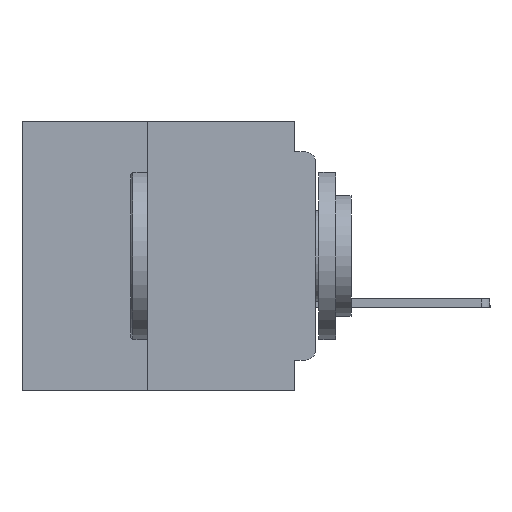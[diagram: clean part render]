
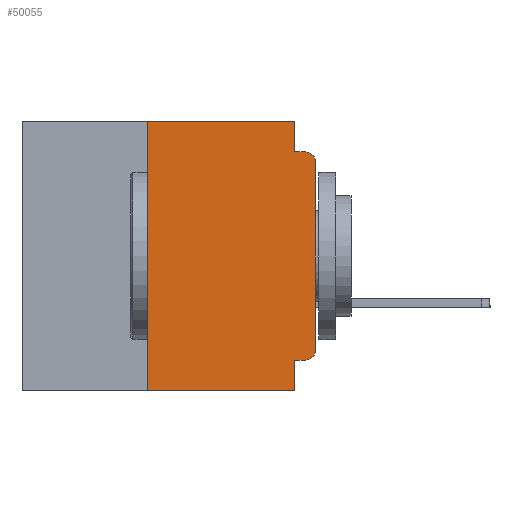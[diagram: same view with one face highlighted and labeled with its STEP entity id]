
A CAD part, left-side view. The second image highlights one B-rep face of the part: STEP entity #50055.
In plain terms, the highlighted planar face has unit normal (-1, 0, 0).
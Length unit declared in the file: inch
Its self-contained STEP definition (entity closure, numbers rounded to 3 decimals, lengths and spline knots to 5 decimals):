
#32 = DIRECTION ( 'NONE',  ( 0., -1., 0. ) ) ;
#233 = CARTESIAN_POINT ( 'NONE',  ( 0., 0.031, -0.4 ) ) ;
#2347 = CARTESIAN_POINT ( 'NONE',  ( 0., 0.437, 0. ) ) ;
#2412 = ORIENTED_EDGE ( 'NONE', *, *, #21963, .F. ) ;
#2658 = VERTEX_POINT ( 'NONE', #31188 ) ;
#2677 = CARTESIAN_POINT ( 'NONE',  ( 0., 0.031, -0.045 ) ) ;
#3046 = CARTESIAN_POINT ( 'NONE',  ( 0., 0.015, -0.355 ) ) ;
#3271 = CARTESIAN_POINT ( 'NONE',  ( 0., 0.437, -0.4 ) ) ;
#3938 = CARTESIAN_POINT ( 'NONE',  ( 0., 0.437, 0. ) ) ;
#4752 = CIRCLE ( 'NONE', #21019, 0.015 ) ;
#5465 = CARTESIAN_POINT ( 'NONE',  ( 0., 0., -0.06 ) ) ;
#7526 = DIRECTION ( 'NONE',  ( 0., -1., 0. ) ) ;
#7736 = CARTESIAN_POINT ( 'NONE',  ( 0., 0.031, 0. ) ) ;
#8598 = EDGE_CURVE ( 'NONE', #13141, #32965, #4752, .T. ) ;
#10267 = DIRECTION ( 'NONE',  ( -1., 0., 0. ) ) ;
#10346 = VECTOR ( 'NONE', #43938, 39.37008 ) ;
#10355 = ORIENTED_EDGE ( 'NONE', *, *, #50103, .F. ) ;
#10613 = ORIENTED_EDGE ( 'NONE', *, *, #42960, .T. ) ;
#11469 = LINE ( 'NONE', #14997, #44432 ) ;
#12647 = ORIENTED_EDGE ( 'NONE', *, *, #53464, .F. ) ;
#12721 = ORIENTED_EDGE ( 'NONE', *, *, #18864, .T. ) ;
#13141 = VERTEX_POINT ( 'NONE', #5465 ) ;
#14222 = VECTOR ( 'NONE', #24063, 39.37008 ) ;
#14935 = LINE ( 'NONE', #7736, #45246 ) ;
#14997 = CARTESIAN_POINT ( 'NONE',  ( 0., 0., 0. ) ) ;
#15523 = VECTOR ( 'NONE', #32, 39.37008 ) ;
#15670 = CARTESIAN_POINT ( 'NONE',  ( 0., 0.031, -0.4 ) ) ;
#16669 = DIRECTION ( 'NONE',  ( 1., 0., 0. ) ) ;
#17147 = DIRECTION ( 'NONE',  ( 0., 0., 1. ) ) ;
#17294 = VERTEX_POINT ( 'NONE', #37693 ) ;
#18864 = EDGE_CURVE ( 'NONE', #2658, #13141, #11469, .T. ) ;
#18992 = VERTEX_POINT ( 'NONE', #19981 ) ;
#19160 = CARTESIAN_POINT ( 'NONE',  ( 0., 0.25, -0.4 ) ) ;
#19406 = CARTESIAN_POINT ( 'NONE',  ( 0., 0.015, -0.06 ) ) ;
#19901 = EDGE_CURVE ( 'NONE', #31632, #17294, #36713, .T. ) ;
#19981 = CARTESIAN_POINT ( 'NONE',  ( 0., 0.031, 0. ) ) ;
#20222 = ORIENTED_EDGE ( 'NONE', *, *, #19901, .F. ) ;
#21019 = AXIS2_PLACEMENT_3D ( 'NONE', #19406, #48093, #23564 ) ;
#21051 = CARTESIAN_POINT ( 'NONE',  ( 0., 0., -0.045 ) ) ;
#21503 = LINE ( 'NONE', #2347, #10346 ) ;
#21934 = VERTEX_POINT ( 'NONE', #19160 ) ;
#21963 = EDGE_CURVE ( 'NONE', #35315, #18992, #21503, .T. ) ;
#23564 = DIRECTION ( 'NONE',  ( 0., 0., -1. ) ) ;
#24063 = DIRECTION ( 'NONE',  ( 0., 0., -1. ) ) ;
#26662 = AXIS2_PLACEMENT_3D ( 'NONE', #3938, #16669, #45443 ) ;
#26748 = ORIENTED_EDGE ( 'NONE', *, *, #34373, .F. ) ;
#30324 = ORIENTED_EDGE ( 'NONE', *, *, #42572, .T. ) ;
#31188 = CARTESIAN_POINT ( 'NONE',  ( 0., 0., -0.34 ) ) ;
#31281 = VECTOR ( 'NONE', #7526, 39.37008 ) ;
#31632 = VERTEX_POINT ( 'NONE', #3046 ) ;
#32727 = DIRECTION ( 'NONE',  ( 0., 0., -1. ) ) ;
#32965 = VERTEX_POINT ( 'NONE', #34492 ) ;
#33181 = VERTEX_POINT ( 'NONE', #2677 ) ;
#34373 = EDGE_CURVE ( 'NONE', #17294, #38753, #37605, .T. ) ;
#34492 = CARTESIAN_POINT ( 'NONE',  ( 0., 0.015, -0.045 ) ) ;
#34685 = LINE ( 'NONE', #45893, #45487 ) ;
#35189 = CARTESIAN_POINT ( 'NONE',  ( 0., 0.015, -0.34 ) ) ;
#35315 = VERTEX_POINT ( 'NONE', #50799 ) ;
#36713 = LINE ( 'NONE', #43071, #46198 ) ;
#37583 = LINE ( 'NONE', #21051, #15523 ) ;
#37605 = LINE ( 'NONE', #15670, #14222 ) ;
#37693 = CARTESIAN_POINT ( 'NONE',  ( 0., 0.031, -0.355 ) ) ;
#38337 = ORIENTED_EDGE ( 'NONE', *, *, #8598, .T. ) ;
#38753 = VERTEX_POINT ( 'NONE', #233 ) ;
#39291 = DIRECTION ( 'NONE',  ( 0., 0., -1. ) ) ;
#39528 = EDGE_LOOP ( 'NONE', ( #12721, #38337, #10355, #12647, #2412, #50643, #30324, #26748, #20222, #10613 ) ) ;
#40884 = LINE ( 'NONE', #3271, #31281 ) ;
#41381 = PLANE ( 'NONE',  #26662 ) ;
#41491 = AXIS2_PLACEMENT_3D ( 'NONE', #35189, #10267, #39291 ) ;
#42572 = EDGE_CURVE ( 'NONE', #21934, #38753, #40884, .T. ) ;
#42960 = EDGE_CURVE ( 'NONE', #31632, #2658, #50893, .T. ) ;
#43071 = CARTESIAN_POINT ( 'NONE',  ( 0., 0., -0.355 ) ) ;
#43869 = DIRECTION ( 'NONE',  ( 0., 0., 1. ) ) ;
#43938 = DIRECTION ( 'NONE',  ( 0., -1., 0. ) ) ;
#44432 = VECTOR ( 'NONE', #43869, 39.37008 ) ;
#45246 = VECTOR ( 'NONE', #32727, 39.37008 ) ;
#45443 = DIRECTION ( 'NONE',  ( 0., 0., -1. ) ) ;
#45487 = VECTOR ( 'NONE', #17147, 39.37008 ) ;
#45893 = CARTESIAN_POINT ( 'NONE',  ( 0., 0.25, -0.4 ) ) ;
#46198 = VECTOR ( 'NONE', #47151, 39.37008 ) ;
#47151 = DIRECTION ( 'NONE',  ( 0., 1., 0. ) ) ;
#48093 = DIRECTION ( 'NONE',  ( -1., 0., 0. ) ) ;
#49629 = FACE_OUTER_BOUND ( 'NONE', #39528, .T. ) ;
#50055 = ADVANCED_FACE ( 'NONE', ( #49629 ), #41381, .F. ) ;
#50103 = EDGE_CURVE ( 'NONE', #33181, #32965, #37583, .T. ) ;
#50643 = ORIENTED_EDGE ( 'NONE', *, *, #50715, .F. ) ;
#50715 = EDGE_CURVE ( 'NONE', #21934, #35315, #34685, .T. ) ;
#50799 = CARTESIAN_POINT ( 'NONE',  ( 0., 0.25, 0. ) ) ;
#50893 = CIRCLE ( 'NONE', #41491, 0.015 ) ;
#53464 = EDGE_CURVE ( 'NONE', #18992, #33181, #14935, .T. ) ;
